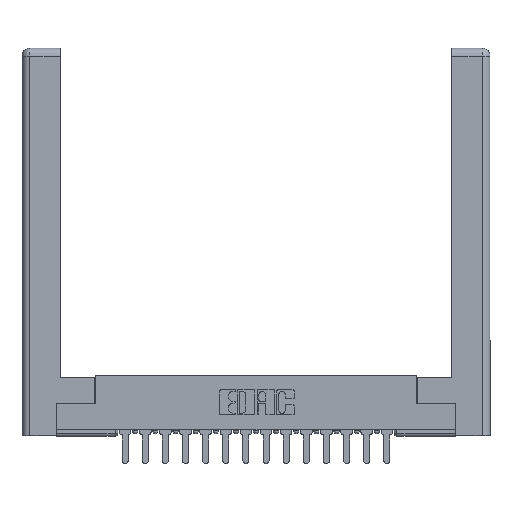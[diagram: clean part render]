
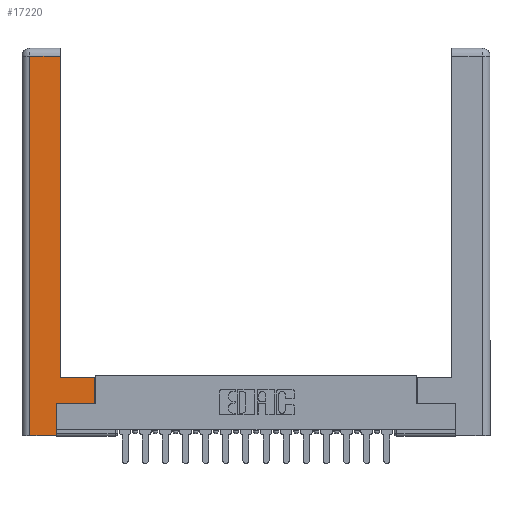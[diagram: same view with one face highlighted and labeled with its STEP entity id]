
A CAD part, top view. The second image highlights one B-rep face of the part: STEP entity #17220.
In plain terms, the highlighted planar face has unit normal (0, 0, 1).
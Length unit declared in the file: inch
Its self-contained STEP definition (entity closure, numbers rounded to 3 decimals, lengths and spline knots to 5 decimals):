
#384 = DIRECTION ( 'NONE',  ( -1., 0., 0. ) ) ;
#519 = CARTESIAN_POINT ( 'NONE',  ( 0.565, 0.245, 0. ) ) ;
#846 = EDGE_LOOP ( 'NONE', ( #18180, #6657, #16384, #5060, #10414, #5690, #12268, #6298 ) ) ;
#955 = AXIS2_PLACEMENT_3D ( 'NONE', #11382, #11157, #2644 ) ;
#1267 = CARTESIAN_POINT ( 'NONE',  ( 0.0615, 2.94, 0. ) ) ;
#1270 = EDGE_CURVE ( 'NONE', #3627, #5004, #8375, .T. ) ;
#1478 = DIRECTION ( 'NONE',  ( 0., -1., 0. ) ) ;
#1521 = VECTOR ( 'NONE', #6711, 39.37008 ) ;
#1759 = VECTOR ( 'NONE', #7737, 39.37008 ) ;
#2183 = VERTEX_POINT ( 'NONE', #15631 ) ;
#2644 = DIRECTION ( 'NONE',  ( -1., 0., 0. ) ) ;
#2840 = CARTESIAN_POINT ( 'NONE',  ( 0.295, 0.45, 0. ) ) ;
#2848 = CARTESIAN_POINT ( 'NONE',  ( 0.0615, 0., 0. ) ) ;
#3176 = VECTOR ( 'NONE', #9177, 39.37008 ) ;
#3214 = CARTESIAN_POINT ( 'NONE',  ( 0.0615, 2.94, 0. ) ) ;
#3627 = VERTEX_POINT ( 'NONE', #10663 ) ;
#3888 = LINE ( 'NONE', #10403, #17524 ) ;
#4204 = EDGE_CURVE ( 'NONE', #15680, #15988, #13161, .T. ) ;
#5004 = VERTEX_POINT ( 'NONE', #2840 ) ;
#5060 = ORIENTED_EDGE ( 'NONE', *, *, #11897, .T. ) ;
#5690 = ORIENTED_EDGE ( 'NONE', *, *, #4204, .T. ) ;
#6298 = ORIENTED_EDGE ( 'NONE', *, *, #1270, .T. ) ;
#6657 = ORIENTED_EDGE ( 'NONE', *, *, #13428, .T. ) ;
#6711 = DIRECTION ( 'NONE',  ( 0., 1., 0. ) ) ;
#6874 = CARTESIAN_POINT ( 'NONE',  ( 0.265, 0., 0. ) ) ;
#6908 = PLANE ( 'NONE',  #955 ) ;
#7294 = DIRECTION ( 'NONE',  ( 0., 1., 0. ) ) ;
#7737 = DIRECTION ( 'NONE',  ( 1., 0., 0. ) ) ;
#8251 = CARTESIAN_POINT ( 'NONE',  ( 0.295, 3., 0. ) ) ;
#8375 = LINE ( 'NONE', #13377, #11065 ) ;
#8807 = LINE ( 'NONE', #3214, #3176 ) ;
#9154 = LINE ( 'NONE', #8251, #1521 ) ;
#9177 = DIRECTION ( 'NONE',  ( -1., 0., 0. ) ) ;
#10403 = CARTESIAN_POINT ( 'NONE',  ( 0.265, 0.245, 0. ) ) ;
#10414 = ORIENTED_EDGE ( 'NONE', *, *, #12845, .T. ) ;
#10663 = CARTESIAN_POINT ( 'NONE',  ( 0.565, 0.45, 0. ) ) ;
#10714 = CARTESIAN_POINT ( 'NONE',  ( 0.565, 0.245, 0. ) ) ;
#11065 = VECTOR ( 'NONE', #384, 39.37008 ) ;
#11157 = DIRECTION ( 'NONE',  ( 0., 0., -1. ) ) ;
#11382 = CARTESIAN_POINT ( 'NONE',  ( 0., 0., 0. ) ) ;
#11504 = VECTOR ( 'NONE', #12773, 39.37008 ) ;
#11897 = EDGE_CURVE ( 'NONE', #16238, #18051, #18137, .T. ) ;
#12268 = ORIENTED_EDGE ( 'NONE', *, *, #12687, .T. ) ;
#12687 = EDGE_CURVE ( 'NONE', #15988, #3627, #13521, .T. ) ;
#12773 = DIRECTION ( 'NONE',  ( 0., 1., 0. ) ) ;
#12845 = EDGE_CURVE ( 'NONE', #18051, #15680, #3888, .T. ) ;
#13161 = LINE ( 'NONE', #519, #1759 ) ;
#13376 = FACE_OUTER_BOUND ( 'NONE', #846, .T. ) ;
#13377 = CARTESIAN_POINT ( 'NONE',  ( 0.295, 0.45, 0. ) ) ;
#13428 = EDGE_CURVE ( 'NONE', #2183, #14482, #8807, .T. ) ;
#13521 = LINE ( 'NONE', #18478, #11504 ) ;
#14321 = VECTOR ( 'NONE', #16619, 39.37008 ) ;
#14482 = VERTEX_POINT ( 'NONE', #1267 ) ;
#14814 = CARTESIAN_POINT ( 'NONE',  ( 0.265, 0., 0. ) ) ;
#15631 = CARTESIAN_POINT ( 'NONE',  ( 0.295, 2.94, 0. ) ) ;
#15680 = VERTEX_POINT ( 'NONE', #18286 ) ;
#15988 = VERTEX_POINT ( 'NONE', #10714 ) ;
#16238 = VERTEX_POINT ( 'NONE', #18130 ) ;
#16384 = ORIENTED_EDGE ( 'NONE', *, *, #16621, .T. ) ;
#16619 = DIRECTION ( 'NONE',  ( 1., 0., 0. ) ) ;
#16621 = EDGE_CURVE ( 'NONE', #14482, #16238, #17402, .T. ) ;
#16989 = EDGE_CURVE ( 'NONE', #5004, #2183, #9154, .T. ) ;
#17220 = ADVANCED_FACE ( 'NONE', ( #13376 ), #6908, .F. ) ;
#17402 = LINE ( 'NONE', #2848, #18323 ) ;
#17524 = VECTOR ( 'NONE', #7294, 39.37008 ) ;
#18051 = VERTEX_POINT ( 'NONE', #14814 ) ;
#18130 = CARTESIAN_POINT ( 'NONE',  ( 0.0615, 0., 0. ) ) ;
#18137 = LINE ( 'NONE', #6874, #14321 ) ;
#18180 = ORIENTED_EDGE ( 'NONE', *, *, #16989, .T. ) ;
#18286 = CARTESIAN_POINT ( 'NONE',  ( 0.265, 0.245, 0. ) ) ;
#18323 = VECTOR ( 'NONE', #1478, 39.37008 ) ;
#18478 = CARTESIAN_POINT ( 'NONE',  ( 0.565, 0.45, 0. ) ) ;
